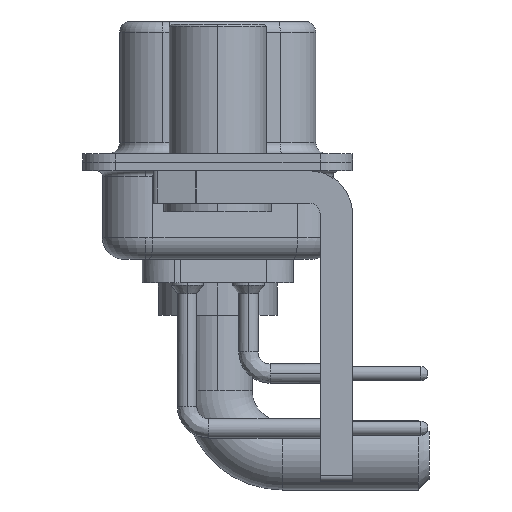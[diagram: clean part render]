
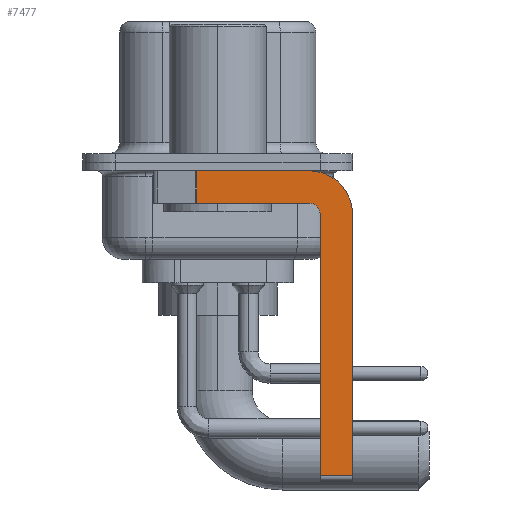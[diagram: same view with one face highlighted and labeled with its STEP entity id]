
A CAD part, left-side view. The second image highlights one B-rep face of the part: STEP entity #7477.
In plain terms, the highlighted planar face has unit normal (-1, 0, 0).
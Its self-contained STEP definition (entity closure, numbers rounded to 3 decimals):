
#517 = VECTOR ( 'NONE', #19702, 1000. ) ;
#550 = CARTESIAN_POINT ( 'NONE',  ( -2.9, -6.25, -14.55 ) ) ;
#564 = AXIS2_PLACEMENT_3D ( 'NONE', #10086, #16868, #16420 ) ;
#1060 = EDGE_CURVE ( 'NONE', #9576, #19587, #12380, .T. ) ;
#1167 = VECTOR ( 'NONE', #6439, 1000. ) ;
#1232 = VECTOR ( 'NONE', #15176, 1000. ) ;
#1236 = EDGE_CURVE ( 'NONE', #1793, #9576, #4095, .T. ) ;
#1793 = VERTEX_POINT ( 'NONE', #2313 ) ;
#2025 = CARTESIAN_POINT ( 'NONE',  ( -2.9, -4.25, -14.55 ) ) ;
#2313 = CARTESIAN_POINT ( 'NONE',  ( -2.9, 0.978, -0.4 ) ) ;
#2746 = ORIENTED_EDGE ( 'NONE', *, *, #14396, .F. ) ;
#2786 = EDGE_CURVE ( 'NONE', #9655, #12342, #21294, .T. ) ;
#2971 = CARTESIAN_POINT ( 'NONE',  ( -2.9, -6.25, -2.4 ) ) ;
#3158 = FACE_OUTER_BOUND ( 'NONE', #12795, .T. ) ;
#3565 = VECTOR ( 'NONE', #12490, 1000. ) ;
#4095 = LINE ( 'NONE', #8951, #3565 ) ;
#4672 = CARTESIAN_POINT ( 'NONE',  ( -2.9, -6.25, -2.4 ) ) ;
#5066 = VECTOR ( 'NONE', #13066, 1000. ) ;
#5362 = EDGE_CURVE ( 'NONE', #1793, #19106, #14731, .T. ) ;
#5457 = ORIENTED_EDGE ( 'NONE', *, *, #12443, .F. ) ;
#5459 = DIRECTION ( 'NONE',  ( 0., 0., 1. ) ) ;
#5676 = ORIENTED_EDGE ( 'NONE', *, *, #6245, .T. ) ;
#6124 = DIRECTION ( 'NONE',  ( 0., 0., 1. ) ) ;
#6245 = EDGE_CURVE ( 'NONE', #9655, #11911, #18725, .T. ) ;
#6326 = CARTESIAN_POINT ( 'NONE',  ( -2.9, 0.978, -1.9 ) ) ;
#6439 = DIRECTION ( 'NONE',  ( 0., 0., -1. ) ) ;
#6717 = ORIENTED_EDGE ( 'NONE', *, *, #1060, .F. ) ;
#7003 = CARTESIAN_POINT ( 'NONE',  ( -2.9, -4.25, -2.4 ) ) ;
#7477 = ADVANCED_FACE ( 'NONE', ( #3158 ), #21841, .F. ) ;
#7564 = DIRECTION ( 'NONE',  ( 1., 0., 0. ) ) ;
#8312 = AXIS2_PLACEMENT_3D ( 'NONE', #7003, #20840, #5459 ) ;
#8951 = CARTESIAN_POINT ( 'NONE',  ( -2.9, 3., -0.4 ) ) ;
#8980 = VERTEX_POINT ( 'NONE', #16993 ) ;
#9576 = VERTEX_POINT ( 'NONE', #16252 ) ;
#9655 = VERTEX_POINT ( 'NONE', #14914 ) ;
#10086 = CARTESIAN_POINT ( 'NONE',  ( -2.9, -4.25, -2.4 ) ) ;
#11361 = CARTESIAN_POINT ( 'NONE',  ( -2.9, 0.978, -1.9 ) ) ;
#11911 = VERTEX_POINT ( 'NONE', #550 ) ;
#12086 = VECTOR ( 'NONE', #6124, 1000. ) ;
#12342 = VERTEX_POINT ( 'NONE', #15744 ) ;
#12380 = CIRCLE ( 'NONE', #20878, 2. ) ;
#12443 = EDGE_CURVE ( 'NONE', #19587, #11911, #19838, .T. ) ;
#12490 = DIRECTION ( 'NONE',  ( 0., -1., 0. ) ) ;
#12795 = EDGE_LOOP ( 'NONE', ( #18244, #19124, #21751, #2746, #14846, #5676, #5457, #6717 ) ) ;
#13066 = DIRECTION ( 'NONE',  ( 0., 0., -1. ) ) ;
#13092 = CARTESIAN_POINT ( 'NONE',  ( -2.9, -4.75, -14.8 ) ) ;
#13223 = EDGE_CURVE ( 'NONE', #8980, #19106, #21367, .T. ) ;
#14396 = EDGE_CURVE ( 'NONE', #12342, #8980, #17857, .T. ) ;
#14731 = LINE ( 'NONE', #6326, #5066 ) ;
#14846 = ORIENTED_EDGE ( 'NONE', *, *, #2786, .F. ) ;
#14914 = CARTESIAN_POINT ( 'NONE',  ( -2.9, -4.75, -14.55 ) ) ;
#14948 = CARTESIAN_POINT ( 'NONE',  ( -2.9, -4.25, -2.4 ) ) ;
#15176 = DIRECTION ( 'NONE',  ( 0., -1., 0. ) ) ;
#15744 = CARTESIAN_POINT ( 'NONE',  ( -2.9, -4.75, -2.4 ) ) ;
#16252 = CARTESIAN_POINT ( 'NONE',  ( -2.9, -4.25, -0.4 ) ) ;
#16420 = DIRECTION ( 'NONE',  ( 0., 0., -1. ) ) ;
#16495 = CARTESIAN_POINT ( 'NONE',  ( -2.9, -4.25, -1.9 ) ) ;
#16868 = DIRECTION ( 'NONE',  ( 1., 0., 0. ) ) ;
#16993 = CARTESIAN_POINT ( 'NONE',  ( -2.9, -4.25, -1.9 ) ) ;
#17857 = CIRCLE ( 'NONE', #8312, 0.5 ) ;
#18244 = ORIENTED_EDGE ( 'NONE', *, *, #1236, .F. ) ;
#18725 = LINE ( 'NONE', #2025, #1232 ) ;
#19106 = VERTEX_POINT ( 'NONE', #11361 ) ;
#19124 = ORIENTED_EDGE ( 'NONE', *, *, #5362, .T. ) ;
#19587 = VERTEX_POINT ( 'NONE', #2971 ) ;
#19702 = DIRECTION ( 'NONE',  ( 0., 1., 0. ) ) ;
#19838 = LINE ( 'NONE', #4672, #1167 ) ;
#20840 = DIRECTION ( 'NONE',  ( -1., 0., 0. ) ) ;
#20878 = AXIS2_PLACEMENT_3D ( 'NONE', #14948, #7564, #21709 ) ;
#21294 = LINE ( 'NONE', #13092, #12086 ) ;
#21367 = LINE ( 'NONE', #16495, #517 ) ;
#21709 = DIRECTION ( 'NONE',  ( 0., 0., -1. ) ) ;
#21751 = ORIENTED_EDGE ( 'NONE', *, *, #13223, .F. ) ;
#21841 = PLANE ( 'NONE',  #564 ) ;
